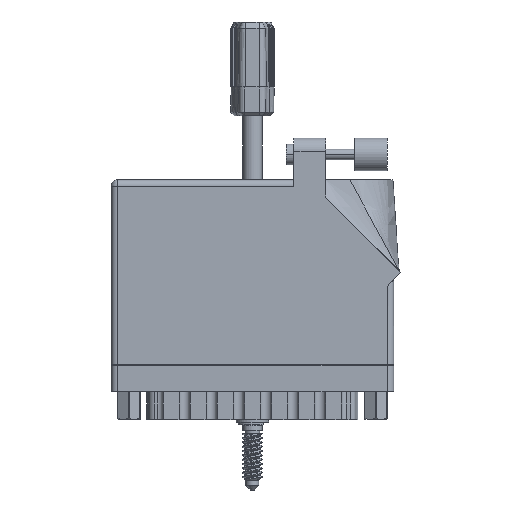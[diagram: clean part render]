
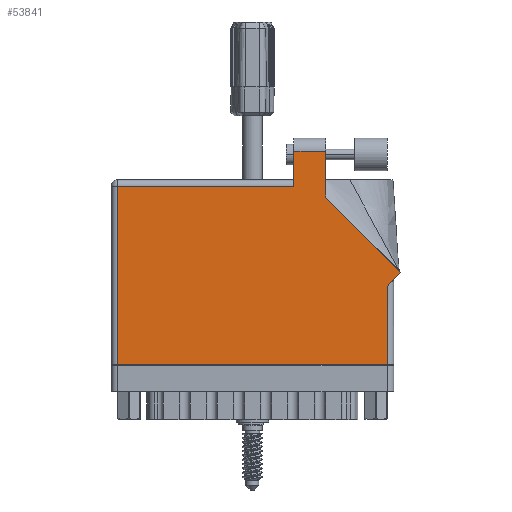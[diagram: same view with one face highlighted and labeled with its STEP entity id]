
A CAD part, front view. The second image highlights one B-rep face of the part: STEP entity #53841.
In plain terms, the highlighted face is planar.
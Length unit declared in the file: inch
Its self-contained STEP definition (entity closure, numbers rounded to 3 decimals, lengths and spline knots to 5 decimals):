
#255 = EDGE_CURVE ( 'NONE', #82601, #79297, #61409, .T. ) ;
#347 = EDGE_CURVE ( 'NONE', #79297, #65783, #15218, .T. ) ;
#2379 = CARTESIAN_POINT ( 'NONE',  ( 1.758, 2.05, 0. ) ) ;
#2572 = CARTESIAN_POINT ( 'NONE',  ( 0., 0., 0. ) ) ;
#3013 = CARTESIAN_POINT ( 'NONE',  ( 1.758, 1.775, 0. ) ) ;
#4810 = CARTESIAN_POINT ( 'NONE',  ( 1.758, 1.713, 0. ) ) ;
#5054 = VECTOR ( 'NONE', #85599, 39.37008 ) ;
#6854 = ORIENTED_EDGE ( 'NONE', *, *, #25642, .T. ) ;
#9981 = DIRECTION ( 'NONE',  ( 0., -1., 0. ) ) ;
#11396 = CARTESIAN_POINT ( 'NONE',  ( 2.656, 0.753, 0. ) ) ;
#11596 = ORIENTED_EDGE ( 'NONE', *, *, #85757, .T. ) ;
#12616 = LINE ( 'NONE', #53158, #38551 ) ;
#15218 = LINE ( 'NONE', #36423, #60312 ) ;
#15575 = DIRECTION ( 'NONE',  ( 1., 0., 0. ) ) ;
#16207 = CARTESIAN_POINT ( 'NONE',  ( 2.78871, 0.88571, 0. ) ) ;
#18321 = VECTOR ( 'NONE', #88569, 39.37008 ) ;
#18581 = PLANE ( 'NONE',  #82144 ) ;
#20674 = ORIENTED_EDGE ( 'NONE', *, *, #347, .T. ) ;
#23662 = VERTEX_POINT ( 'NONE', #41219 ) ;
#25642 = EDGE_CURVE ( 'NONE', #27345, #51590, #56653, .T. ) ;
#27075 = FACE_OUTER_BOUND ( 'NONE', #77365, .T. ) ;
#27345 = VERTEX_POINT ( 'NONE', #29682 ) ;
#27428 = VERTEX_POINT ( 'NONE', #11396 ) ;
#28633 = EDGE_CURVE ( 'NONE', #45051, #82601, #30189, .T. ) ;
#29664 = ORIENTED_EDGE ( 'NONE', *, *, #92033, .T. ) ;
#29682 = CARTESIAN_POINT ( 'NONE',  ( 2.065, 1.60942, 0. ) ) ;
#30189 = LINE ( 'NONE', #3013, #56119 ) ;
#30419 = VERTEX_POINT ( 'NONE', #89282 ) ;
#33854 = CARTESIAN_POINT ( 'NONE',  ( 1.758, 2.05, 0. ) ) ;
#36423 = CARTESIAN_POINT ( 'NONE',  ( 0.062, 0., 0. ) ) ;
#36612 = CARTESIAN_POINT ( 'NONE',  ( 2.656, 0.815, 0. ) ) ;
#37605 = DIRECTION ( 'NONE',  ( -0.707, 0.707, 0. ) ) ;
#37931 = LINE ( 'NONE', #2379, #85300 ) ;
#38551 = VECTOR ( 'NONE', #60112, 39.37008 ) ;
#40647 = CARTESIAN_POINT ( 'NONE',  ( 0.062, 1.713, 0. ) ) ;
#41219 = CARTESIAN_POINT ( 'NONE',  ( 2.78871, 0.88571, 0. ) ) ;
#45051 = VERTEX_POINT ( 'NONE', #33854 ) ;
#46062 = DIRECTION ( 'NONE',  ( 0., 0., -1. ) ) ;
#50258 = EDGE_CURVE ( 'NONE', #51590, #45051, #37931, .T. ) ;
#51590 = VERTEX_POINT ( 'NONE', #52533 ) ;
#52533 = CARTESIAN_POINT ( 'NONE',  ( 2.065, 2.05, 0. ) ) ;
#52806 = DIRECTION ( 'NONE',  ( -1., 0., 0. ) ) ;
#53158 = CARTESIAN_POINT ( 'NONE',  ( 2.718, 0.815, 0. ) ) ;
#53841 = ADVANCED_FACE ( 'NONE', ( #27075 ), #18581, .F. ) ;
#56119 = VECTOR ( 'NONE', #9981, 39.37008 ) ;
#56432 = EDGE_CURVE ( 'NONE', #27428, #23662, #12616, .T. ) ;
#56622 = CARTESIAN_POINT ( 'NONE',  ( 0., 1.713, 0. ) ) ;
#56653 = LINE ( 'NONE', #81283, #18321 ) ;
#56942 = ORIENTED_EDGE ( 'NONE', *, *, #255, .T. ) ;
#58513 = DIRECTION ( 'NONE',  ( 0., -1., 0. ) ) ;
#58978 = VECTOR ( 'NONE', #37605, 39.37008 ) ;
#59271 = ORIENTED_EDGE ( 'NONE', *, *, #56432, .T. ) ;
#60058 = ORIENTED_EDGE ( 'NONE', *, *, #50258, .T. ) ;
#60112 = DIRECTION ( 'NONE',  ( 0.707, 0.707, 0. ) ) ;
#60312 = VECTOR ( 'NONE', #58513, 39.37008 ) ;
#61140 = VECTOR ( 'NONE', #15575, 39.37008 ) ;
#61409 = LINE ( 'NONE', #56622, #5054 ) ;
#65783 = VERTEX_POINT ( 'NONE', #71063 ) ;
#71063 = CARTESIAN_POINT ( 'NONE',  ( 0.062, 0., 0. ) ) ;
#72524 = LINE ( 'NONE', #16207, #58978 ) ;
#75738 = LINE ( 'NONE', #2572, #61140 ) ;
#77365 = EDGE_LOOP ( 'NONE', ( #6854, #60058, #81572, #56942, #20674, #89803, #29664, #59271, #11596 ) ) ;
#77666 = EDGE_CURVE ( 'NONE', #65783, #30419, #75738, .T. ) ;
#79297 = VERTEX_POINT ( 'NONE', #40647 ) ;
#81283 = CARTESIAN_POINT ( 'NONE',  ( 2.065, 1.60942, 0. ) ) ;
#81572 = ORIENTED_EDGE ( 'NONE', *, *, #28633, .T. ) ;
#81676 = DIRECTION ( 'NONE',  ( -1., 0., 0. ) ) ;
#82088 = CARTESIAN_POINT ( 'NONE',  ( 0., 1.775, 0. ) ) ;
#82144 = AXIS2_PLACEMENT_3D ( 'NONE', #82088, #46062, #81676 ) ;
#82601 = VERTEX_POINT ( 'NONE', #4810 ) ;
#82749 = VECTOR ( 'NONE', #87975, 39.37008 ) ;
#85300 = VECTOR ( 'NONE', #52806, 39.37008 ) ;
#85599 = DIRECTION ( 'NONE',  ( -1., 0., 0. ) ) ;
#85757 = EDGE_CURVE ( 'NONE', #23662, #27345, #72524, .T. ) ;
#87975 = DIRECTION ( 'NONE',  ( 0., 1., 0. ) ) ;
#88569 = DIRECTION ( 'NONE',  ( 0., 1., 0. ) ) ;
#89282 = CARTESIAN_POINT ( 'NONE',  ( 2.656, 0., 0. ) ) ;
#89573 = LINE ( 'NONE', #36612, #82749 ) ;
#89803 = ORIENTED_EDGE ( 'NONE', *, *, #77666, .T. ) ;
#92033 = EDGE_CURVE ( 'NONE', #30419, #27428, #89573, .T. ) ;
